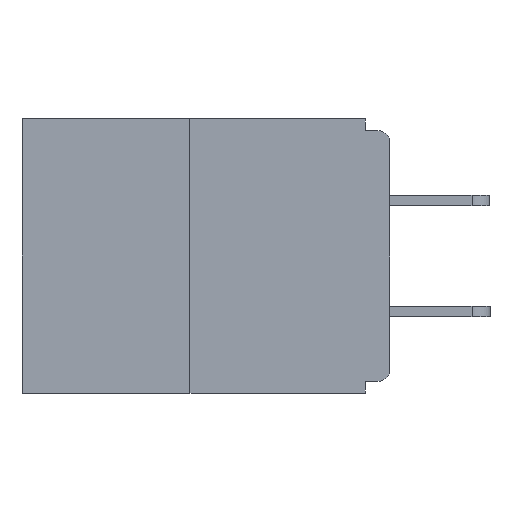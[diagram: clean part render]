
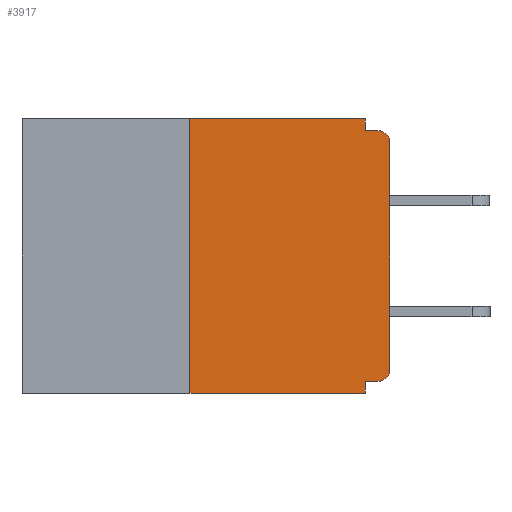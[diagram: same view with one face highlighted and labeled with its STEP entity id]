
A CAD part, left-side view. The second image highlights one B-rep face of the part: STEP entity #3917.
In plain terms, the highlighted planar face has unit normal (-1, 0, 0).
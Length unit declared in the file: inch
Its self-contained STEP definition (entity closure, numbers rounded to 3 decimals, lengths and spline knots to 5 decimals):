
#86 = DIRECTION ( 'NONE',  ( 0., 0., 1. ) ) ;
#402 = EDGE_CURVE ( 'NONE', #3573, #6869, #2788, .T. ) ;
#461 = CARTESIAN_POINT ( 'NONE',  ( 0., 0.015, -0.015 ) ) ;
#715 = VECTOR ( 'NONE', #8154, 39.37008 ) ;
#807 = CARTESIAN_POINT ( 'NONE',  ( 0., 0.46, 0. ) ) ;
#993 = VECTOR ( 'NONE', #9350, 39.37008 ) ;
#1304 = VERTEX_POINT ( 'NONE', #3132 ) ;
#1489 = CARTESIAN_POINT ( 'NONE',  ( 0., 0.46, 0. ) ) ;
#1492 = LINE ( 'NONE', #8564, #10549 ) ;
#1778 = ORIENTED_EDGE ( 'NONE', *, *, #11267, .F. ) ;
#1871 = ORIENTED_EDGE ( 'NONE', *, *, #5421, .T. ) ;
#1873 = CARTESIAN_POINT ( 'NONE',  ( 0., 0.031, -0.015 ) ) ;
#2123 = DIRECTION ( 'NONE',  ( 0., 0., -1. ) ) ;
#2138 = DIRECTION ( 'NONE',  ( 0., 1., 0. ) ) ;
#2386 = CARTESIAN_POINT ( 'NONE',  ( 0., 0.015, -0.313 ) ) ;
#2414 = ORIENTED_EDGE ( 'NONE', *, *, #9969, .T. ) ;
#2582 = ORIENTED_EDGE ( 'NONE', *, *, #3592, .F. ) ;
#2788 = LINE ( 'NONE', #5557, #5857 ) ;
#2864 = CARTESIAN_POINT ( 'NONE',  ( 0., 0., -0.015 ) ) ;
#3116 = CARTESIAN_POINT ( 'NONE',  ( 0., 0., -0.328 ) ) ;
#3132 = CARTESIAN_POINT ( 'NONE',  ( 0., 0.031, -0.343 ) ) ;
#3250 = VECTOR ( 'NONE', #2138, 39.37008 ) ;
#3567 = VERTEX_POINT ( 'NONE', #12547 ) ;
#3573 = VERTEX_POINT ( 'NONE', #7077 ) ;
#3592 = EDGE_CURVE ( 'NONE', #6869, #13215, #13632, .T. ) ;
#3899 = CARTESIAN_POINT ( 'NONE',  ( 0., 0.031, -0.343 ) ) ;
#3917 = ADVANCED_FACE ( 'NONE', ( #5923 ), #12681, .F. ) ;
#4267 = VERTEX_POINT ( 'NONE', #8431 ) ;
#4324 = CARTESIAN_POINT ( 'NONE',  ( 0., 0.015, -0.03 ) ) ;
#4349 = CARTESIAN_POINT ( 'NONE',  ( 0., 0., -0.313 ) ) ;
#4945 = VECTOR ( 'NONE', #5151, 39.37008 ) ;
#5052 = ORIENTED_EDGE ( 'NONE', *, *, #402, .F. ) ;
#5122 = LINE ( 'NONE', #2864, #4945 ) ;
#5151 = DIRECTION ( 'NONE',  ( 0., -1., 0. ) ) ;
#5357 = EDGE_CURVE ( 'NONE', #3567, #11372, #8220, .T. ) ;
#5421 = EDGE_CURVE ( 'NONE', #3567, #7070, #12133, .T. ) ;
#5466 = ORIENTED_EDGE ( 'NONE', *, *, #5538, .F. ) ;
#5538 = EDGE_CURVE ( 'NONE', #6050, #12976, #5122, .T. ) ;
#5557 = CARTESIAN_POINT ( 'NONE',  ( 0., 0.25, 0. ) ) ;
#5857 = VECTOR ( 'NONE', #86, 39.37008 ) ;
#5869 = CIRCLE ( 'NONE', #9229, 0.015 ) ;
#5923 = FACE_OUTER_BOUND ( 'NONE', #13645, .T. ) ;
#6050 = VERTEX_POINT ( 'NONE', #1873 ) ;
#6162 = DIRECTION ( 'NONE',  ( 0., 0., -1. ) ) ;
#6279 = EDGE_CURVE ( 'NONE', #7070, #4267, #7328, .T. ) ;
#6494 = DIRECTION ( 'NONE',  ( 0., 0., 1. ) ) ;
#6763 = ORIENTED_EDGE ( 'NONE', *, *, #5357, .F. ) ;
#6869 = VERTEX_POINT ( 'NONE', #10497 ) ;
#6879 = AXIS2_PLACEMENT_3D ( 'NONE', #807, #10610, #6162 ) ;
#7070 = VERTEX_POINT ( 'NONE', #4349 ) ;
#7077 = CARTESIAN_POINT ( 'NONE',  ( 0., 0.25, -0.343 ) ) ;
#7163 = EDGE_CURVE ( 'NONE', #3573, #1304, #7180, .T. ) ;
#7180 = LINE ( 'NONE', #9513, #10593 ) ;
#7235 = DIRECTION ( 'NONE',  ( 0., -1., 0. ) ) ;
#7328 = LINE ( 'NONE', #10803, #11938 ) ;
#8154 = DIRECTION ( 'NONE',  ( 0., -1., 0. ) ) ;
#8220 = LINE ( 'NONE', #3116, #3250 ) ;
#8337 = EDGE_CURVE ( 'NONE', #13215, #6050, #1492, .T. ) ;
#8431 = CARTESIAN_POINT ( 'NONE',  ( 0., 0., -0.03 ) ) ;
#8564 = CARTESIAN_POINT ( 'NONE',  ( 0., 0.031, 0. ) ) ;
#9229 = AXIS2_PLACEMENT_3D ( 'NONE', #4324, #12053, #11974 ) ;
#9350 = DIRECTION ( 'NONE',  ( 0., 0., -1. ) ) ;
#9513 = CARTESIAN_POINT ( 'NONE',  ( 0., 0.46, -0.343 ) ) ;
#9823 = LINE ( 'NONE', #3899, #993 ) ;
#9969 = EDGE_CURVE ( 'NONE', #4267, #12976, #5869, .T. ) ;
#10031 = DIRECTION ( 'NONE',  ( -1., 0., 0. ) ) ;
#10155 = DIRECTION ( 'NONE',  ( 0., 0., -1. ) ) ;
#10497 = CARTESIAN_POINT ( 'NONE',  ( 0., 0.25, 0. ) ) ;
#10549 = VECTOR ( 'NONE', #2123, 39.37008 ) ;
#10593 = VECTOR ( 'NONE', #7235, 39.37008 ) ;
#10597 = CARTESIAN_POINT ( 'NONE',  ( 0., 0.031, -0.328 ) ) ;
#10610 = DIRECTION ( 'NONE',  ( 1., 0., 0. ) ) ;
#10803 = CARTESIAN_POINT ( 'NONE',  ( 0., 0., 0. ) ) ;
#11267 = EDGE_CURVE ( 'NONE', #11372, #1304, #9823, .T. ) ;
#11372 = VERTEX_POINT ( 'NONE', #10597 ) ;
#11640 = CARTESIAN_POINT ( 'NONE',  ( 0., 0.031, 0. ) ) ;
#11668 = AXIS2_PLACEMENT_3D ( 'NONE', #2386, #10031, #10155 ) ;
#11938 = VECTOR ( 'NONE', #6494, 39.37008 ) ;
#11974 = DIRECTION ( 'NONE',  ( 0., 0., -1. ) ) ;
#12053 = DIRECTION ( 'NONE',  ( -1., 0., 0. ) ) ;
#12133 = CIRCLE ( 'NONE', #11668, 0.015 ) ;
#12197 = ORIENTED_EDGE ( 'NONE', *, *, #6279, .T. ) ;
#12547 = CARTESIAN_POINT ( 'NONE',  ( 0., 0.015, -0.328 ) ) ;
#12681 = PLANE ( 'NONE',  #6879 ) ;
#12976 = VERTEX_POINT ( 'NONE', #461 ) ;
#13215 = VERTEX_POINT ( 'NONE', #11640 ) ;
#13632 = LINE ( 'NONE', #1489, #715 ) ;
#13645 = EDGE_LOOP ( 'NONE', ( #2582, #5052, #13854, #1778, #6763, #1871, #12197, #2414, #5466, #13814 ) ) ;
#13814 = ORIENTED_EDGE ( 'NONE', *, *, #8337, .F. ) ;
#13854 = ORIENTED_EDGE ( 'NONE', *, *, #7163, .T. ) ;
